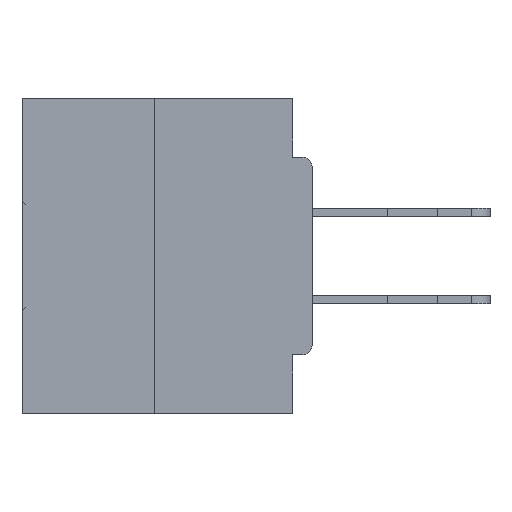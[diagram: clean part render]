
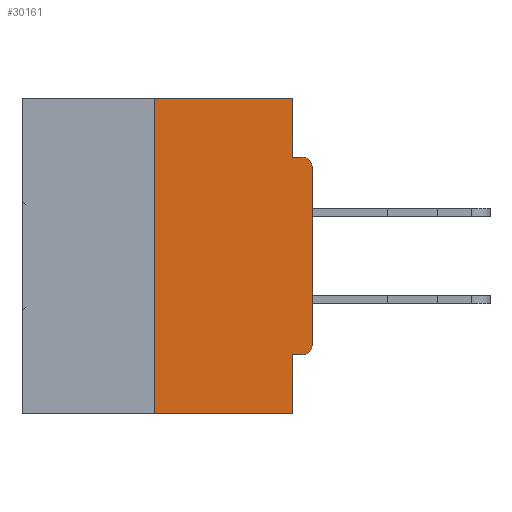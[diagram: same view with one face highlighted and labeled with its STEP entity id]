
A CAD part, left-side view. The second image highlights one B-rep face of the part: STEP entity #30161.
In plain terms, the highlighted planar face has unit normal (-1, 0, 0).
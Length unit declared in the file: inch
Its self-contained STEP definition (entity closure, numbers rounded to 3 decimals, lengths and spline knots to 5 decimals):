
#1 = EDGE_CURVE ( 'NONE', #6872, #21985, #32847, .T. ) ;
#350 = EDGE_CURVE ( 'NONE', #21496, #34537, #2636, .T. ) ;
#1960 = CARTESIAN_POINT ( 'NONE',  ( 0., 0., 0. ) ) ;
#2636 = LINE ( 'NONE', #29091, #9986 ) ;
#2710 = LINE ( 'NONE', #1960, #15682 ) ;
#3869 = CARTESIAN_POINT ( 'NONE',  ( 0., 0.015, -0.1085 ) ) ;
#5488 = CIRCLE ( 'NONE', #23000, 0.015 ) ;
#5901 = DIRECTION ( 'NONE',  ( 0., 0., -1. ) ) ;
#5905 = CARTESIAN_POINT ( 'NONE',  ( 0., 0.46, 0. ) ) ;
#6116 = CARTESIAN_POINT ( 'NONE',  ( 0., 0., -0.1085 ) ) ;
#6720 = EDGE_CURVE ( 'NONE', #21639, #21985, #5488, .T. ) ;
#6872 = VERTEX_POINT ( 'NONE', #14165 ) ;
#7121 = EDGE_CURVE ( 'NONE', #34537, #18276, #25715, .T. ) ;
#8635 = LINE ( 'NONE', #26834, #39747 ) ;
#9401 = EDGE_CURVE ( 'NONE', #11944, #18276, #15923, .T. ) ;
#9986 = VECTOR ( 'NONE', #41733, 39.37008 ) ;
#11107 = ORIENTED_EDGE ( 'NONE', *, *, #28058, .F. ) ;
#11944 = VERTEX_POINT ( 'NONE', #22905 ) ;
#12502 = DIRECTION ( 'NONE',  ( 0., 0., -1. ) ) ;
#13766 = ORIENTED_EDGE ( 'NONE', *, *, #32915, .F. ) ;
#13874 = CARTESIAN_POINT ( 'NONE',  ( 0., 0.25, 0. ) ) ;
#14165 = CARTESIAN_POINT ( 'NONE',  ( 0., 0.031, -0.0935 ) ) ;
#14457 = CARTESIAN_POINT ( 'NONE',  ( 0., 0.031, -0.5 ) ) ;
#15682 = VECTOR ( 'NONE', #25176, 39.37008 ) ;
#15923 = LINE ( 'NONE', #26034, #27426 ) ;
#16265 = CARTESIAN_POINT ( 'NONE',  ( 0., 0.031, -0.4065 ) ) ;
#16484 = DIRECTION ( 'NONE',  ( 0., 0., 1. ) ) ;
#16893 = VECTOR ( 'NONE', #21665, 39.37008 ) ;
#17317 = VERTEX_POINT ( 'NONE', #32228 ) ;
#18276 = VERTEX_POINT ( 'NONE', #14457 ) ;
#18283 = CARTESIAN_POINT ( 'NONE',  ( 0., 0.031, -0.5 ) ) ;
#19846 = EDGE_CURVE ( 'NONE', #21496, #17317, #21342, .T. ) ;
#20095 = DIRECTION ( 'NONE',  ( 0., 0., -1. ) ) ;
#21342 = CIRCLE ( 'NONE', #42026, 0.015 ) ;
#21474 = EDGE_CURVE ( 'NONE', #17317, #21639, #2710, .T. ) ;
#21496 = VERTEX_POINT ( 'NONE', #21986 ) ;
#21639 = VERTEX_POINT ( 'NONE', #6116 ) ;
#21665 = DIRECTION ( 'NONE',  ( 0., 0., -1. ) ) ;
#21985 = VERTEX_POINT ( 'NONE', #24955 ) ;
#21986 = CARTESIAN_POINT ( 'NONE',  ( 0., 0.015, -0.4065 ) ) ;
#22335 = LINE ( 'NONE', #5905, #30728 ) ;
#22440 = VECTOR ( 'NONE', #39181, 39.37008 ) ;
#22905 = CARTESIAN_POINT ( 'NONE',  ( 0., 0.25, -0.5 ) ) ;
#23000 = AXIS2_PLACEMENT_3D ( 'NONE', #3869, #36997, #40163 ) ;
#23453 = ORIENTED_EDGE ( 'NONE', *, *, #19846, .T. ) ;
#23706 = ORIENTED_EDGE ( 'NONE', *, *, #21474, .T. ) ;
#24788 = PLANE ( 'NONE',  #39533 ) ;
#24955 = CARTESIAN_POINT ( 'NONE',  ( 0., 0.015, -0.0935 ) ) ;
#25176 = DIRECTION ( 'NONE',  ( 0., 0., 1. ) ) ;
#25439 = EDGE_CURVE ( 'NONE', #11944, #35639, #8635, .T. ) ;
#25591 = ORIENTED_EDGE ( 'NONE', *, *, #6720, .T. ) ;
#25715 = LINE ( 'NONE', #18283, #16893 ) ;
#25775 = DIRECTION ( 'NONE',  ( 1., 0., 0. ) ) ;
#26034 = CARTESIAN_POINT ( 'NONE',  ( 0., 0.46, -0.5 ) ) ;
#26455 = CARTESIAN_POINT ( 'NONE',  ( 0., 0.031, 0. ) ) ;
#26834 = CARTESIAN_POINT ( 'NONE',  ( 0., 0.25, 0. ) ) ;
#27426 = VECTOR ( 'NONE', #39511, 39.37008 ) ;
#28058 = EDGE_CURVE ( 'NONE', #31427, #6872, #39916, .T. ) ;
#28767 = CARTESIAN_POINT ( 'NONE',  ( 0., 0., -0.0935 ) ) ;
#29091 = CARTESIAN_POINT ( 'NONE',  ( 0., 0., -0.4065 ) ) ;
#30161 = ADVANCED_FACE ( 'NONE', ( #38741 ), #24788, .F. ) ;
#30586 = VECTOR ( 'NONE', #20095, 39.37008 ) ;
#30728 = VECTOR ( 'NONE', #32633, 39.37008 ) ;
#31427 = VERTEX_POINT ( 'NONE', #26455 ) ;
#32228 = CARTESIAN_POINT ( 'NONE',  ( 0., 0., -0.3915 ) ) ;
#32633 = DIRECTION ( 'NONE',  ( 0., -1., 0. ) ) ;
#32847 = LINE ( 'NONE', #28767, #22440 ) ;
#32915 = EDGE_CURVE ( 'NONE', #35639, #31427, #22335, .T. ) ;
#34537 = VERTEX_POINT ( 'NONE', #16265 ) ;
#34863 = ORIENTED_EDGE ( 'NONE', *, *, #350, .F. ) ;
#35633 = CARTESIAN_POINT ( 'NONE',  ( 0., 0.015, -0.3915 ) ) ;
#35639 = VERTEX_POINT ( 'NONE', #13874 ) ;
#36837 = ORIENTED_EDGE ( 'NONE', *, *, #25439, .F. ) ;
#36997 = DIRECTION ( 'NONE',  ( -1., 0., 0. ) ) ;
#38562 = CARTESIAN_POINT ( 'NONE',  ( 0., 0.46, 0. ) ) ;
#38708 = ORIENTED_EDGE ( 'NONE', *, *, #9401, .T. ) ;
#38741 = FACE_OUTER_BOUND ( 'NONE', #42645, .T. ) ;
#38932 = DIRECTION ( 'NONE',  ( -1., 0., 0. ) ) ;
#39060 = ORIENTED_EDGE ( 'NONE', *, *, #7121, .F. ) ;
#39181 = DIRECTION ( 'NONE',  ( 0., -1., 0. ) ) ;
#39511 = DIRECTION ( 'NONE',  ( 0., -1., 0. ) ) ;
#39533 = AXIS2_PLACEMENT_3D ( 'NONE', #38562, #25775, #5901 ) ;
#39747 = VECTOR ( 'NONE', #16484, 39.37008 ) ;
#39916 = LINE ( 'NONE', #40121, #30586 ) ;
#40121 = CARTESIAN_POINT ( 'NONE',  ( 0., 0.031, 0. ) ) ;
#40163 = DIRECTION ( 'NONE',  ( 0., 0., -1. ) ) ;
#41733 = DIRECTION ( 'NONE',  ( 0., 1., 0. ) ) ;
#41748 = ORIENTED_EDGE ( 'NONE', *, *, #1, .F. ) ;
#42026 = AXIS2_PLACEMENT_3D ( 'NONE', #35633, #38932, #12502 ) ;
#42645 = EDGE_LOOP ( 'NONE', ( #13766, #36837, #38708, #39060, #34863, #23453, #23706, #25591, #41748, #11107 ) ) ;
